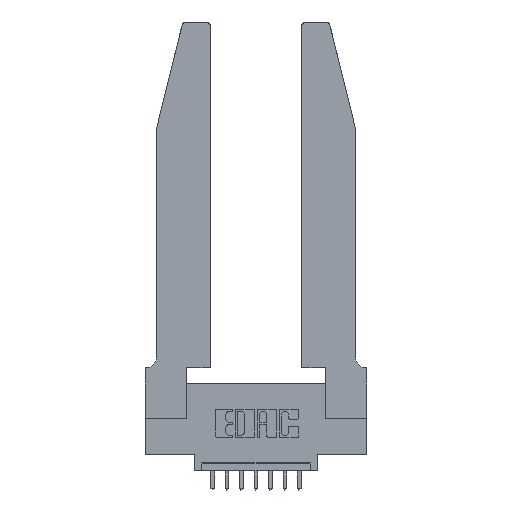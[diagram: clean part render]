
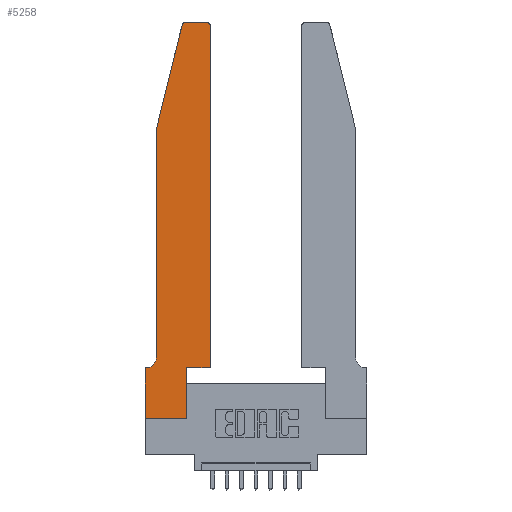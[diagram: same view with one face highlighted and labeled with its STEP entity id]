
A CAD part, top view. The second image highlights one B-rep face of the part: STEP entity #5258.
In plain terms, the highlighted planar face has unit normal (0, 0, 1).
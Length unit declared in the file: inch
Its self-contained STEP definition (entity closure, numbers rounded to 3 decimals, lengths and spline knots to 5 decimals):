
#17 = VECTOR ( 'NONE', #3745, 39.37008 ) ;
#50 = VECTOR ( 'NONE', #13513, 39.37008 ) ;
#141 = CARTESIAN_POINT ( 'NONE',  ( 0.0755, 2., 0.37 ) ) ;
#694 = EDGE_CURVE ( 'NONE', #9756, #2648, #12196, .T. ) ;
#787 = LINE ( 'NONE', #5965, #6555 ) ;
#833 = CARTESIAN_POINT ( 'NONE',  ( 0.0055, 0.42, 0.37 ) ) ;
#1032 = DIRECTION ( 'NONE',  ( 0., 1., 0. ) ) ;
#1183 = DIRECTION ( 'NONE',  ( 0., -1., 0. ) ) ;
#1197 = VECTOR ( 'NONE', #8534, 39.37008 ) ;
#1234 = DIRECTION ( 'NONE',  ( 1., 0., 0. ) ) ;
#1412 = CARTESIAN_POINT ( 'NONE',  ( 0.0755, 0.35, 0.37 ) ) ;
#1486 = DIRECTION ( 'NONE',  ( -0.239, -0.971, 0. ) ) ;
#1526 = VERTEX_POINT ( 'NONE', #4457 ) ;
#1572 = AXIS2_PLACEMENT_3D ( 'NONE', #3263, #11314, #6790 ) ;
#1862 = LINE ( 'NONE', #6655, #50 ) ;
#1908 = DIRECTION ( 'NONE',  ( 0., 0., 1. ) ) ;
#2209 = VERTEX_POINT ( 'NONE', #11599 ) ;
#2300 = CARTESIAN_POINT ( 'NONE',  ( 0., 0.35, 0.37 ) ) ;
#2362 = VECTOR ( 'NONE', #12751, 39.37008 ) ;
#2445 = ORIENTED_EDGE ( 'NONE', *, *, #8904, .T. ) ;
#2604 = CARTESIAN_POINT ( 'NONE',  ( 0., 0., 0.37 ) ) ;
#2608 = CARTESIAN_POINT ( 'NONE',  ( 0.0755, 2., 0.37 ) ) ;
#2648 = VERTEX_POINT ( 'NONE', #2779 ) ;
#2779 = CARTESIAN_POINT ( 'NONE',  ( 0.4205, 2.75, 0.37 ) ) ;
#3252 = AXIS2_PLACEMENT_3D ( 'NONE', #2300, #11444, #1234 ) ;
#3263 = CARTESIAN_POINT ( 'NONE',  ( 0.4205, 2.72, 0.37 ) ) ;
#3288 = EDGE_CURVE ( 'NONE', #6303, #12523, #787, .T. ) ;
#3340 = CARTESIAN_POINT ( 'NONE',  ( 0.4505, 0.35, 0.37 ) ) ;
#3522 = FACE_OUTER_BOUND ( 'NONE', #8396, .T. ) ;
#3595 = VECTOR ( 'NONE', #1486, 39.37008 ) ;
#3689 = VECTOR ( 'NONE', #5851, 39.37008 ) ;
#3745 = DIRECTION ( 'NONE',  ( 1., 0., 0. ) ) ;
#3751 = CARTESIAN_POINT ( 'NONE',  ( 0.284, 2.75, 0.37 ) ) ;
#3836 = CARTESIAN_POINT ( 'NONE',  ( 0.4505, 2.72, 0.37 ) ) ;
#4457 = CARTESIAN_POINT ( 'NONE',  ( 0.0755, 0.42, 0.37 ) ) ;
#4770 = VERTEX_POINT ( 'NONE', #6295 ) ;
#4826 = EDGE_CURVE ( 'NONE', #10623, #2209, #14302, .T. ) ;
#4977 = VECTOR ( 'NONE', #1032, 39.37008 ) ;
#5014 = VERTEX_POINT ( 'NONE', #141 ) ;
#5151 = LINE ( 'NONE', #3340, #4977 ) ;
#5258 = ADVANCED_FACE ( 'NONE', ( #3522 ), #5829, .T. ) ;
#5320 = EDGE_CURVE ( 'NONE', #4770, #9756, #5151, .T. ) ;
#5645 = CARTESIAN_POINT ( 'NONE',  ( 0.0755, 2., 0.37 ) ) ;
#5829 = PLANE ( 'NONE',  #3252 ) ;
#5836 = EDGE_CURVE ( 'NONE', #5014, #1526, #11787, .T. ) ;
#5851 = DIRECTION ( 'NONE',  ( 0., -1., 0. ) ) ;
#5965 = CARTESIAN_POINT ( 'NONE',  ( 0., 0., 0.37 ) ) ;
#6295 = CARTESIAN_POINT ( 'NONE',  ( 0.4505, 0.35, 0.37 ) ) ;
#6303 = VERTEX_POINT ( 'NONE', #6671 ) ;
#6322 = CARTESIAN_POINT ( 'NONE',  ( 0.2605, 2.75, 0.37 ) ) ;
#6328 = LINE ( 'NONE', #2604, #17 ) ;
#6555 = VECTOR ( 'NONE', #1183, 39.37008 ) ;
#6578 = DIRECTION ( 'NONE',  ( -1., 0., 0. ) ) ;
#6655 = CARTESIAN_POINT ( 'NONE',  ( 0.4505, 0.35, 0.37 ) ) ;
#6671 = CARTESIAN_POINT ( 'NONE',  ( 0., 0.35, 0.37 ) ) ;
#6707 = EDGE_CURVE ( 'NONE', #2209, #4770, #1862, .T. ) ;
#6790 = DIRECTION ( 'NONE',  ( 1., 0., 0. ) ) ;
#7137 = CARTESIAN_POINT ( 'NONE',  ( 0., 0., 0.37 ) ) ;
#7223 = ORIENTED_EDGE ( 'NONE', *, *, #11181, .T. ) ;
#7509 = ORIENTED_EDGE ( 'NONE', *, *, #694, .T. ) ;
#7548 = ORIENTED_EDGE ( 'NONE', *, *, #5836, .T. ) ;
#7583 = ORIENTED_EDGE ( 'NONE', *, *, #3288, .T. ) ;
#7651 = CARTESIAN_POINT ( 'NONE',  ( 0.25487, 2.72718, 0.37 ) ) ;
#7709 = EDGE_CURVE ( 'NONE', #12523, #10623, #6328, .T. ) ;
#7874 = AXIS2_PLACEMENT_3D ( 'NONE', #12212, #1908, #14456 ) ;
#7896 = VERTEX_POINT ( 'NONE', #7651 ) ;
#8260 = LINE ( 'NONE', #6322, #8777 ) ;
#8396 = EDGE_LOOP ( 'NONE', ( #7223, #13060, #11167, #7548, #2445, #11833, #7583, #8463, #14592, #12837, #14885, #7509 ) ) ;
#8463 = ORIENTED_EDGE ( 'NONE', *, *, #7709, .T. ) ;
#8490 = LINE ( 'NONE', #1412, #2362 ) ;
#8534 = DIRECTION ( 'NONE',  ( 0., 1., 0. ) ) ;
#8598 = EDGE_CURVE ( 'NONE', #10928, #6303, #8490, .T. ) ;
#8777 = VECTOR ( 'NONE', #13273, 39.37008 ) ;
#8904 = EDGE_CURVE ( 'NONE', #1526, #10928, #13274, .T. ) ;
#9164 = EDGE_CURVE ( 'NONE', #7896, #5014, #10095, .T. ) ;
#9756 = VERTEX_POINT ( 'NONE', #3836 ) ;
#10095 = LINE ( 'NONE', #2608, #3595 ) ;
#10623 = VERTEX_POINT ( 'NONE', #13436 ) ;
#10624 = EDGE_CURVE ( 'NONE', #11057, #7896, #13943, .T. ) ;
#10928 = VERTEX_POINT ( 'NONE', #11553 ) ;
#10952 = CARTESIAN_POINT ( 'NONE',  ( 0.2865, 0.35, 0.37 ) ) ;
#11057 = VERTEX_POINT ( 'NONE', #3751 ) ;
#11167 = ORIENTED_EDGE ( 'NONE', *, *, #9164, .T. ) ;
#11181 = EDGE_CURVE ( 'NONE', #2648, #11057, #8260, .T. ) ;
#11314 = DIRECTION ( 'NONE',  ( 0., 0., 1. ) ) ;
#11444 = DIRECTION ( 'NONE',  ( 0., 0., 1. ) ) ;
#11553 = CARTESIAN_POINT ( 'NONE',  ( 0.0055, 0.35, 0.37 ) ) ;
#11599 = CARTESIAN_POINT ( 'NONE',  ( 0.2865, 0.35, 0.37 ) ) ;
#11787 = LINE ( 'NONE', #5645, #3689 ) ;
#11833 = ORIENTED_EDGE ( 'NONE', *, *, #8598, .T. ) ;
#12196 = CIRCLE ( 'NONE', #1572, 0.03 ) ;
#12212 = CARTESIAN_POINT ( 'NONE',  ( 0.284, 2.72, 0.37 ) ) ;
#12523 = VERTEX_POINT ( 'NONE', #7137 ) ;
#12751 = DIRECTION ( 'NONE',  ( -1., 0., 0. ) ) ;
#12837 = ORIENTED_EDGE ( 'NONE', *, *, #6707, .T. ) ;
#13060 = ORIENTED_EDGE ( 'NONE', *, *, #10624, .T. ) ;
#13273 = DIRECTION ( 'NONE',  ( -1., 0., 0. ) ) ;
#13274 = CIRCLE ( 'NONE', #13478, 0.07 ) ;
#13436 = CARTESIAN_POINT ( 'NONE',  ( 0.2865, 0., 0.37 ) ) ;
#13478 = AXIS2_PLACEMENT_3D ( 'NONE', #833, #14651, #6578 ) ;
#13513 = DIRECTION ( 'NONE',  ( 1., 0., 0. ) ) ;
#13943 = CIRCLE ( 'NONE', #7874, 0.03 ) ;
#14302 = LINE ( 'NONE', #10952, #1197 ) ;
#14456 = DIRECTION ( 'NONE',  ( 1., 0., 0. ) ) ;
#14592 = ORIENTED_EDGE ( 'NONE', *, *, #4826, .T. ) ;
#14651 = DIRECTION ( 'NONE',  ( 0., 0., -1. ) ) ;
#14885 = ORIENTED_EDGE ( 'NONE', *, *, #5320, .T. ) ;
